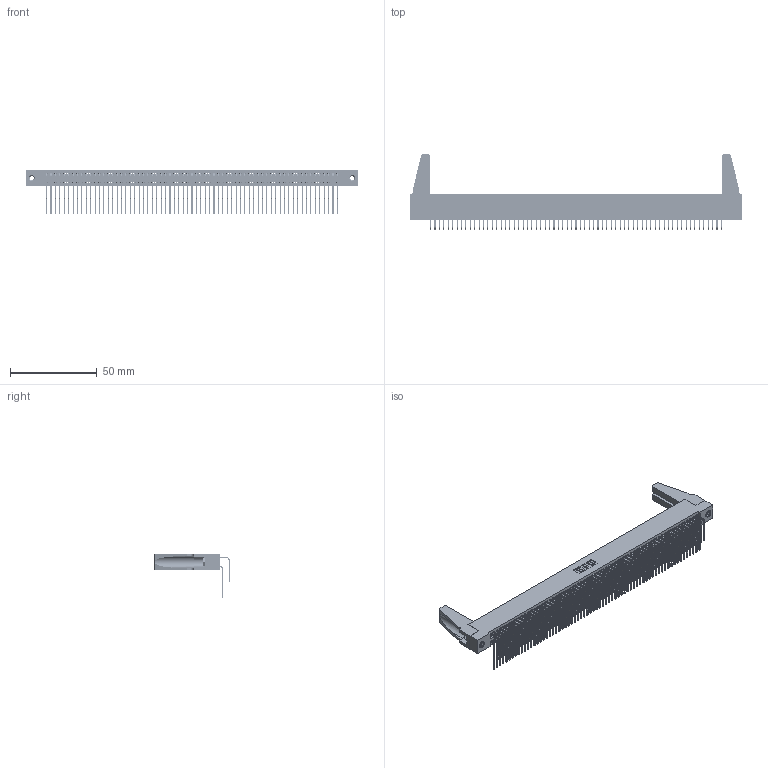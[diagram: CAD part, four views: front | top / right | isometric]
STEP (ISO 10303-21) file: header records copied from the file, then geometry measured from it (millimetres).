
FILE_DESCRIPTION (( 'STEP AP203' ), '1' );
FILE_NAME ('395-134-559-288.STEP', '2019-10-29T14:06:37', ( '' ), ( '' ), 'SwSTEP 2.0', 'SolidWorks 2016', '' );
FILE_SCHEMA (( 'CONFIG_CONTROL_DESIGN' ));
Length unit declared in the file: inch
Products named in the file (6): 345-292-001_559 Tail - 2; 345 Part_Flush Mounting Lugs - 0.156 Dia-TH; 345-250-001_345-250-001-102; 345-220-078_345-220-088; 395-134-559-288; 345-292-001_558 559 Tail - 1
Assembly tree (139 placements, depth 2):
  395-134-559-288
    345 Part_Flush Mounting Lugs - 0.156 Dia-TH
    345-292-001_558 559 Tail - 1  x67
    345-292-001_559 Tail - 2  x67
    345-250-001_345-250-001-102  x2
    345-220-078_345-220-088  x2
Bounding box: 191.41 x 43.42 x 25.53 mm (x, y, z)
Volume: 22851.7 mm3; surface area: 36212.3 mm2
Topology: 139 solids, 139 shells, 7218 faces, 21425 edges, 14094 vertices
Faces by surface type: plane 4842, cylinder 2360, cone 12, torus 4
Entity records: 53004 total; most frequent: CARTESIAN_POINT 8901, ORIENTED_EDGE 8744, DIRECTION 7796, EDGE_CURVE 4372, LINE 3890, VECTOR 3890, VERTEX_POINT 2906, AXIS2_PLACEMENT_3D 1953
